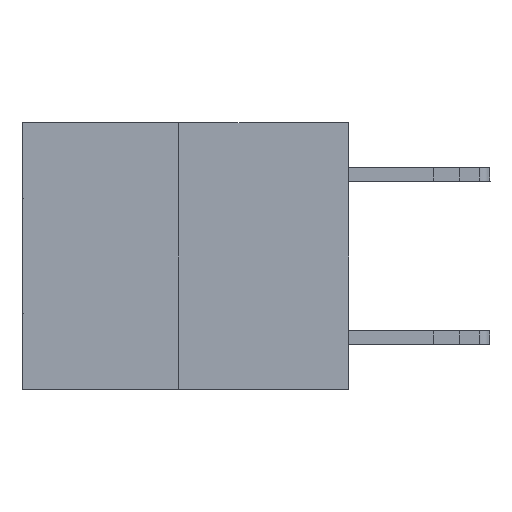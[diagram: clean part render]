
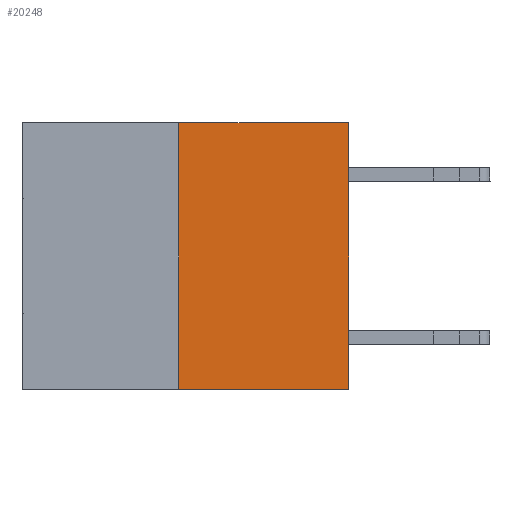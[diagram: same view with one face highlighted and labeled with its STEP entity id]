
A CAD part, left-side view. The second image highlights one B-rep face of the part: STEP entity #20248.
In plain terms, the highlighted planar face has unit normal (-1, 0, 0).
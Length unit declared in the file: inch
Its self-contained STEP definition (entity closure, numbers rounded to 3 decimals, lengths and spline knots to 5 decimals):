
#628 = LINE ( 'NONE', #28917, #2188 ) ;
#2022 = ORIENTED_EDGE ( 'NONE', *, *, #16060, .F. ) ;
#2188 = VECTOR ( 'NONE', #16089, 39.37008 ) ;
#4536 = EDGE_CURVE ( 'NONE', #6523, #10113, #16737, .T. ) ;
#5074 = ORIENTED_EDGE ( 'NONE', *, *, #4536, .T. ) ;
#5787 = DIRECTION ( 'NONE',  ( 0., -1., 0. ) ) ;
#6523 = VERTEX_POINT ( 'NONE', #23014 ) ;
#8420 = CARTESIAN_POINT ( 'NONE',  ( 0., 0.312, 0. ) ) ;
#8938 = EDGE_CURVE ( 'NONE', #10427, #6523, #22801, .T. ) ;
#10113 = VERTEX_POINT ( 'NONE', #20111 ) ;
#10427 = VERTEX_POINT ( 'NONE', #24765 ) ;
#11500 = AXIS2_PLACEMENT_3D ( 'NONE', #31675, #31980, #32089 ) ;
#12784 = LINE ( 'NONE', #19036, #32218 ) ;
#14343 = DIRECTION ( 'NONE',  ( 0., -1., 0. ) ) ;
#15852 = PLANE ( 'NONE',  #11500 ) ;
#16060 = EDGE_CURVE ( 'NONE', #10427, #25767, #628, .T. ) ;
#16089 = DIRECTION ( 'NONE',  ( 0., 0., 1. ) ) ;
#16737 = LINE ( 'NONE', #17501, #22674 ) ;
#17501 = CARTESIAN_POINT ( 'NONE',  ( 0., 0., 0. ) ) ;
#19036 = CARTESIAN_POINT ( 'NONE',  ( 0., 0.6, 0. ) ) ;
#20111 = CARTESIAN_POINT ( 'NONE',  ( 0., 0., 0. ) ) ;
#20248 = ADVANCED_FACE ( 'NONE', ( #24496 ), #15852, .F. ) ;
#20925 = CARTESIAN_POINT ( 'NONE',  ( 0., 0.6, -0.49 ) ) ;
#21982 = VECTOR ( 'NONE', #5787, 39.37008 ) ;
#22674 = VECTOR ( 'NONE', #25236, 39.37008 ) ;
#22801 = LINE ( 'NONE', #20925, #21982 ) ;
#23014 = CARTESIAN_POINT ( 'NONE',  ( 0., 0., -0.49 ) ) ;
#24496 = FACE_OUTER_BOUND ( 'NONE', #31359, .T. ) ;
#24765 = CARTESIAN_POINT ( 'NONE',  ( 0., 0.312, -0.49 ) ) ;
#25236 = DIRECTION ( 'NONE',  ( 0., 0., 1. ) ) ;
#25767 = VERTEX_POINT ( 'NONE', #8420 ) ;
#28917 = CARTESIAN_POINT ( 'NONE',  ( 0., 0.312, -0.49 ) ) ;
#29235 = EDGE_CURVE ( 'NONE', #25767, #10113, #12784, .T. ) ;
#30152 = ORIENTED_EDGE ( 'NONE', *, *, #8938, .T. ) ;
#31359 = EDGE_LOOP ( 'NONE', ( #2022, #30152, #5074, #31524 ) ) ;
#31524 = ORIENTED_EDGE ( 'NONE', *, *, #29235, .F. ) ;
#31675 = CARTESIAN_POINT ( 'NONE',  ( 0., 0.6, 0. ) ) ;
#31980 = DIRECTION ( 'NONE',  ( 1., 0., 0. ) ) ;
#32089 = DIRECTION ( 'NONE',  ( 0., 0., -1. ) ) ;
#32218 = VECTOR ( 'NONE', #14343, 39.37008 ) ;
